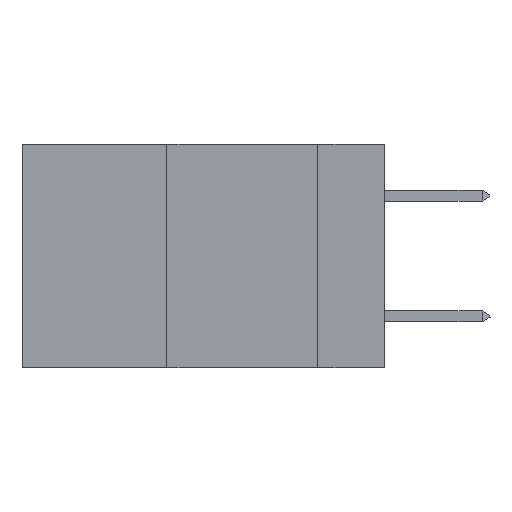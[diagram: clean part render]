
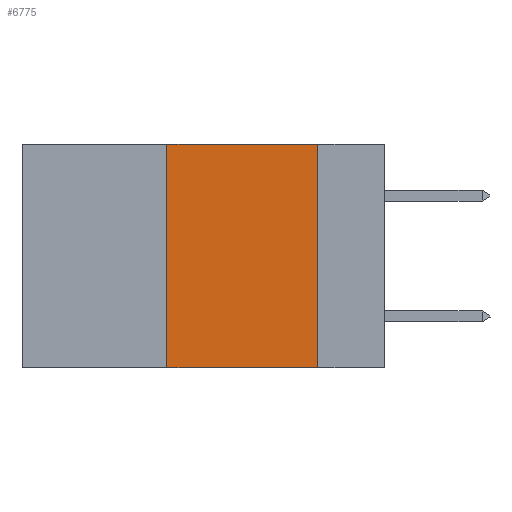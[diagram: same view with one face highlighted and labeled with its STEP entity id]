
A CAD part, left-side view. The second image highlights one B-rep face of the part: STEP entity #6775.
In plain terms, the highlighted planar face has unit normal (-1, 0, 0).
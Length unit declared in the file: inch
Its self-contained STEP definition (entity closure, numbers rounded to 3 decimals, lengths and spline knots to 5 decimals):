
#3 = VERTEX_POINT ( 'NONE', #6594 ) ;
#236 = LINE ( 'NONE', #8023, #6322 ) ;
#497 = EDGE_CURVE ( 'NONE', #8494, #3, #1966, .T. ) ;
#1554 = DIRECTION ( 'NONE',  ( 0., -1., 0. ) ) ;
#1966 = LINE ( 'NONE', #7615, #11946 ) ;
#3451 = ORIENTED_EDGE ( 'NONE', *, *, #497, .F. ) ;
#4319 = VERTEX_POINT ( 'NONE', #11087 ) ;
#5260 = FACE_OUTER_BOUND ( 'NONE', #13573, .T. ) ;
#5362 = EDGE_CURVE ( 'NONE', #11552, #8494, #236, .T. ) ;
#5971 = DIRECTION ( 'NONE',  ( 0., -1., 0. ) ) ;
#6231 = LINE ( 'NONE', #13819, #8470 ) ;
#6322 = VECTOR ( 'NONE', #1554, 39.37008 ) ;
#6594 = CARTESIAN_POINT ( 'NONE',  ( 0., 0.11, -0.37 ) ) ;
#6775 = ADVANCED_FACE ( 'NONE', ( #5260 ), #13945, .F. ) ;
#7615 = CARTESIAN_POINT ( 'NONE',  ( 0., 0.11, 0. ) ) ;
#8023 = CARTESIAN_POINT ( 'NONE',  ( 0., 0.6, 0. ) ) ;
#8470 = VECTOR ( 'NONE', #5971, 39.37008 ) ;
#8494 = VERTEX_POINT ( 'NONE', #10478 ) ;
#8746 = DIRECTION ( 'NONE',  ( 0., 0., -1. ) ) ;
#8874 = EDGE_CURVE ( 'NONE', #4319, #3, #6231, .T. ) ;
#9222 = LINE ( 'NONE', #11027, #12298 ) ;
#10478 = CARTESIAN_POINT ( 'NONE',  ( 0., 0.11, 0. ) ) ;
#10741 = EDGE_CURVE ( 'NONE', #4319, #11552, #9222, .T. ) ;
#11027 = CARTESIAN_POINT ( 'NONE',  ( 0., 0.36, 0. ) ) ;
#11087 = CARTESIAN_POINT ( 'NONE',  ( 0., 0.36, -0.37 ) ) ;
#11319 = CARTESIAN_POINT ( 'NONE',  ( 0., 0.6, 0. ) ) ;
#11552 = VERTEX_POINT ( 'NONE', #16569 ) ;
#11946 = VECTOR ( 'NONE', #15422, 39.37008 ) ;
#12298 = VECTOR ( 'NONE', #13660, 39.37008 ) ;
#13573 = EDGE_LOOP ( 'NONE', ( #3451, #15496, #15303, #16743 ) ) ;
#13660 = DIRECTION ( 'NONE',  ( 0., 0., 1. ) ) ;
#13819 = CARTESIAN_POINT ( 'NONE',  ( 0., 0.6, -0.37 ) ) ;
#13945 = PLANE ( 'NONE',  #15494 ) ;
#15303 = ORIENTED_EDGE ( 'NONE', *, *, #10741, .F. ) ;
#15422 = DIRECTION ( 'NONE',  ( 0., 0., -1. ) ) ;
#15494 = AXIS2_PLACEMENT_3D ( 'NONE', #11319, #16552, #8746 ) ;
#15496 = ORIENTED_EDGE ( 'NONE', *, *, #5362, .F. ) ;
#16552 = DIRECTION ( 'NONE',  ( 1., 0., 0. ) ) ;
#16569 = CARTESIAN_POINT ( 'NONE',  ( 0., 0.36, 0. ) ) ;
#16743 = ORIENTED_EDGE ( 'NONE', *, *, #8874, .T. ) ;
